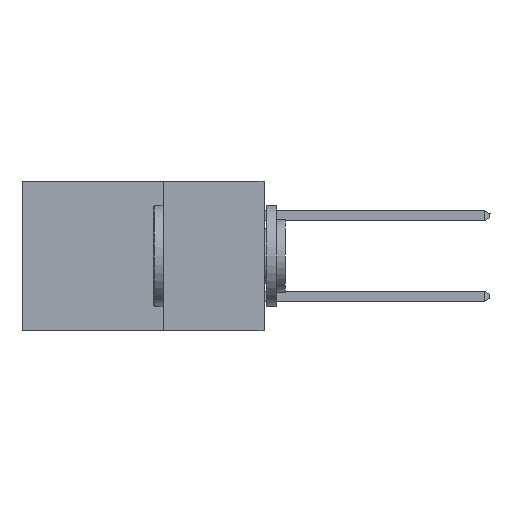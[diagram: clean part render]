
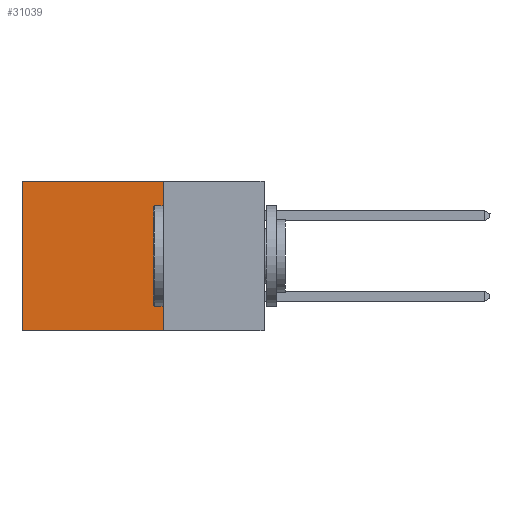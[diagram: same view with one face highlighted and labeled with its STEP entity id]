
A CAD part, left-side view. The second image highlights one B-rep face of the part: STEP entity #31039.
In plain terms, the highlighted planar face has unit normal (-1, 0, 0).
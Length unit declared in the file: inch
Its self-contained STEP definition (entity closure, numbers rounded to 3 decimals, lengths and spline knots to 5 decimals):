
#122 = EDGE_CURVE ( 'NONE', #18523, #23794, #10555, .T. ) ;
#471 = FACE_OUTER_BOUND ( 'NONE', #19426, .T. ) ;
#1385 = LINE ( 'NONE', #29896, #27929 ) ;
#2432 = ORIENTED_EDGE ( 'NONE', *, *, #29689, .F. ) ;
#3727 = VECTOR ( 'NONE', #18927, 39.37008 ) ;
#5572 = CARTESIAN_POINT ( 'NONE',  ( 0.298, 0.6, 0. ) ) ;
#6077 = EDGE_CURVE ( 'NONE', #18523, #24177, #14037, .T. ) ;
#6211 = CARTESIAN_POINT ( 'NONE',  ( 0.298, 0.25, 0. ) ) ;
#6709 = ORIENTED_EDGE ( 'NONE', *, *, #6077, .T. ) ;
#6904 = VERTEX_POINT ( 'NONE', #9872 ) ;
#8582 = VECTOR ( 'NONE', #26145, 39.37008 ) ;
#9377 = LINE ( 'NONE', #5572, #8582 ) ;
#9872 = CARTESIAN_POINT ( 'NONE',  ( 0.298, 0.6, -0.37 ) ) ;
#10555 = LINE ( 'NONE', #18897, #3727 ) ;
#13678 = DIRECTION ( 'NONE',  ( 1., 0., 0. ) ) ;
#14028 = ORIENTED_EDGE ( 'NONE', *, *, #122, .F. ) ;
#14037 = LINE ( 'NONE', #6211, #19251 ) ;
#14087 = DIRECTION ( 'NONE',  ( 0., 1., 0. ) ) ;
#14135 = EDGE_CURVE ( 'NONE', #24177, #6904, #9377, .T. ) ;
#17118 = DIRECTION ( 'NONE',  ( 0., 1., 0. ) ) ;
#18314 = CARTESIAN_POINT ( 'NONE',  ( 0.298, 0.25, -0.37 ) ) ;
#18523 = VERTEX_POINT ( 'NONE', #26679 ) ;
#18897 = CARTESIAN_POINT ( 'NONE',  ( 0.298, 0.25, 0. ) ) ;
#18927 = DIRECTION ( 'NONE',  ( 0., 0., -1. ) ) ;
#19251 = VECTOR ( 'NONE', #14087, 39.37008 ) ;
#19426 = EDGE_LOOP ( 'NONE', ( #26164, #2432, #14028, #6709 ) ) ;
#23794 = VERTEX_POINT ( 'NONE', #18314 ) ;
#23906 = CARTESIAN_POINT ( 'NONE',  ( 0.298, 0.25, 0. ) ) ;
#24177 = VERTEX_POINT ( 'NONE', #24620 ) ;
#24620 = CARTESIAN_POINT ( 'NONE',  ( 0.298, 0.6, 0. ) ) ;
#24712 = AXIS2_PLACEMENT_3D ( 'NONE', #23906, #13678, #31613 ) ;
#26145 = DIRECTION ( 'NONE',  ( 0., 0., -1. ) ) ;
#26164 = ORIENTED_EDGE ( 'NONE', *, *, #14135, .T. ) ;
#26370 = PLANE ( 'NONE',  #24712 ) ;
#26679 = CARTESIAN_POINT ( 'NONE',  ( 0.298, 0.25, 0. ) ) ;
#27929 = VECTOR ( 'NONE', #17118, 39.37008 ) ;
#29689 = EDGE_CURVE ( 'NONE', #23794, #6904, #1385, .T. ) ;
#29896 = CARTESIAN_POINT ( 'NONE',  ( 0.298, 0.25, -0.37 ) ) ;
#31039 = ADVANCED_FACE ( 'NONE', ( #471 ), #26370, .F. ) ;
#31613 = DIRECTION ( 'NONE',  ( 0., 0., -1. ) ) ;
